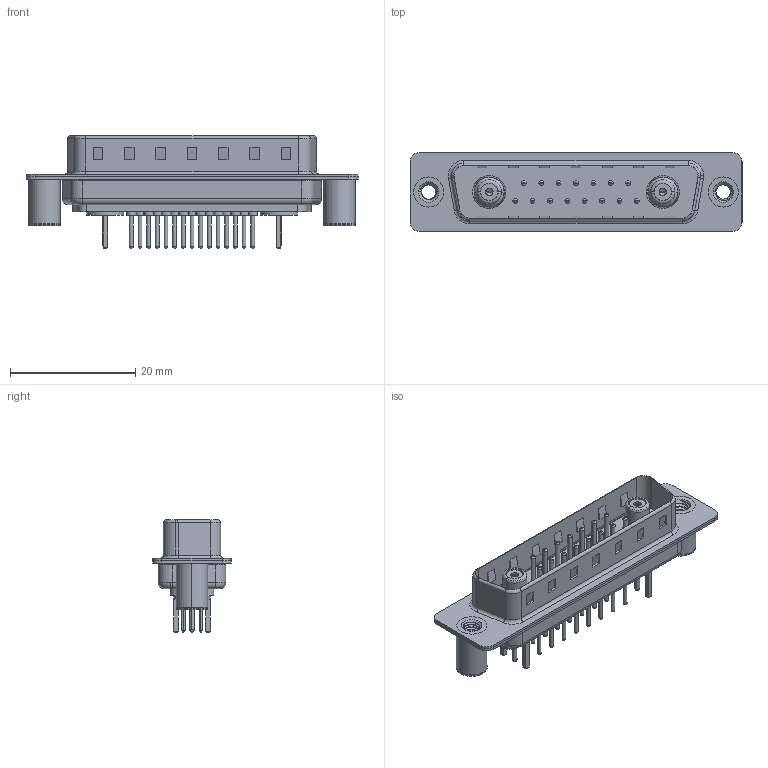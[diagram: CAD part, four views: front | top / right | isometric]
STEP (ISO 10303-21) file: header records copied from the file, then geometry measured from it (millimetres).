
FILE_DESCRIPTION (( 'STEP AP203' ), '1' );
FILE_NAME ('627-17W2624-5TB.STEP', '2019-05-27T23:10:16', ( '' ), ( '' ), 'SwSTEP 2.0', 'SolidWorks 2016', '' );
FILE_SCHEMA (( 'CONFIG_CONTROL_DESIGN' ));
Length unit declared in the file: millimetre
Products named in the file (14): Co-Ax Jack_Straight PC Tail; 627Combo Threaded Board Spacer_3; Locking Collar; Co-Ax Jack Assy_S; 627Combo Shell Rear_25 Contacts; 627Combo Contact Row 1_24; 627Combo Contact Row 2_24; Socket_Str; 627Combo Threaded Board Spacer_B; 627Combo Housing_17W2; Insulator Socket; 627-17W2624-5TB; Insulator Socket 2; 627Combo Shell Front_25 Contacts
Assembly tree (27 placements, depth 3):
  627-17W2624-5TB
    627Combo Housing_17W2
    627Combo Shell Rear_25 Contacts
    627Combo Shell Front_25 Contacts
    627Combo Threaded Board Spacer_B
    Co-Ax Jack Assy_S  x2
      Co-Ax Jack_Straight PC Tail
      Insulator Socket
      Insulator Socket 2
      Locking Collar
      Socket_Str
    627Combo Threaded Board Spacer_3
    627Combo Contact Row 1_24  x7
    627Combo Contact Row 2_24  x8
Bounding box: 53 x 12.6 x 17.9 mm (x, y, z)
Volume: 2886.2 mm3; surface area: 7853.6 mm2
Topology: 30 solids, 30 shells, 1191 faces, 2660 edges, 1631 vertices
Faces by surface type: cylinder 469, plane 370, torus 302, cone 36, bspline 10, sphere 4
Entity records: 26178 total; most frequent: CARTESIAN_POINT 7383, DIRECTION 3764, ORIENTED_EDGE 3378, EDGE_CURVE 1689, AXIS2_PLACEMENT_3D 1474, VERTEX_POINT 1067, EDGE_LOOP 854, VECTOR 816
